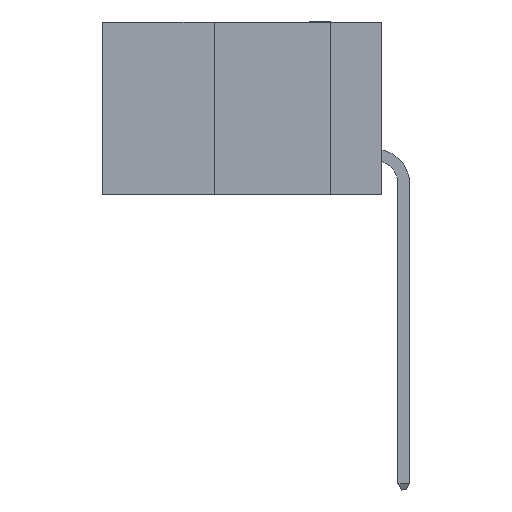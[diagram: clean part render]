
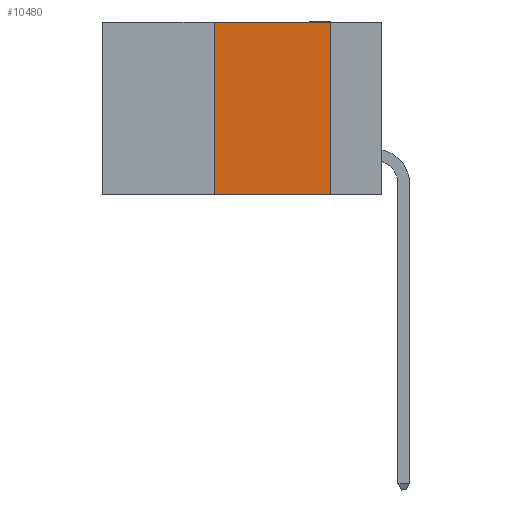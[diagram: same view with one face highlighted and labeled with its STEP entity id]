
A CAD part, left-side view. The second image highlights one B-rep face of the part: STEP entity #10480.
In plain terms, the highlighted planar face has unit normal (-1, 0, 0).
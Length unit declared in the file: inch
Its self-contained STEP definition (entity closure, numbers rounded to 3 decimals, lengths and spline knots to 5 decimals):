
#11 = ORIENTED_EDGE ( 'NONE', *, *, #4980, .F. ) ;
#479 = ORIENTED_EDGE ( 'NONE', *, *, #6891, .F. ) ;
#1325 = EDGE_CURVE ( 'NONE', #3748, #7478, #6699, .T. ) ;
#3245 = DIRECTION ( 'NONE',  ( 0., 0., -1. ) ) ;
#3409 = CARTESIAN_POINT ( 'NONE',  ( 0., 0.6, 0. ) ) ;
#3561 = CARTESIAN_POINT ( 'NONE',  ( 0., 0.11, 0. ) ) ;
#3644 = FACE_OUTER_BOUND ( 'NONE', #9182, .T. ) ;
#3748 = VERTEX_POINT ( 'NONE', #10097 ) ;
#4023 = VECTOR ( 'NONE', #10777, 39.37008 ) ;
#4320 = DIRECTION ( 'NONE',  ( 0., -1., 0. ) ) ;
#4980 = EDGE_CURVE ( 'NONE', #5077, #5996, #14956, .T. ) ;
#5077 = VERTEX_POINT ( 'NONE', #14675 ) ;
#5645 = LINE ( 'NONE', #6619, #14918 ) ;
#5758 = DIRECTION ( 'NONE',  ( 1., 0., 0. ) ) ;
#5996 = VERTEX_POINT ( 'NONE', #6702 ) ;
#6239 = VECTOR ( 'NONE', #14519, 39.37008 ) ;
#6619 = CARTESIAN_POINT ( 'NONE',  ( 0., 0.6, 0. ) ) ;
#6699 = LINE ( 'NONE', #3561, #4023 ) ;
#6702 = CARTESIAN_POINT ( 'NONE',  ( 0., 0.36, 0. ) ) ;
#6750 = CARTESIAN_POINT ( 'NONE',  ( 0., 0.11, -0.37 ) ) ;
#6891 = EDGE_CURVE ( 'NONE', #5996, #3748, #5645, .T. ) ;
#7478 = VERTEX_POINT ( 'NONE', #6750 ) ;
#7846 = CARTESIAN_POINT ( 'NONE',  ( 0., 0.6, -0.37 ) ) ;
#8190 = LINE ( 'NONE', #7846, #8388 ) ;
#8388 = VECTOR ( 'NONE', #10204, 39.37008 ) ;
#9182 = EDGE_LOOP ( 'NONE', ( #15441, #479, #11, #15531 ) ) ;
#10097 = CARTESIAN_POINT ( 'NONE',  ( 0., 0.11, 0. ) ) ;
#10204 = DIRECTION ( 'NONE',  ( 0., -1., 0. ) ) ;
#10480 = ADVANCED_FACE ( 'NONE', ( #3644 ), #10643, .F. ) ;
#10643 = PLANE ( 'NONE',  #12958 ) ;
#10777 = DIRECTION ( 'NONE',  ( 0., 0., -1. ) ) ;
#12958 = AXIS2_PLACEMENT_3D ( 'NONE', #3409, #5758, #3245 ) ;
#13322 = CARTESIAN_POINT ( 'NONE',  ( 0., 0.36, 0. ) ) ;
#14519 = DIRECTION ( 'NONE',  ( 0., 0., 1. ) ) ;
#14675 = CARTESIAN_POINT ( 'NONE',  ( 0., 0.36, -0.37 ) ) ;
#14918 = VECTOR ( 'NONE', #4320, 39.37008 ) ;
#14956 = LINE ( 'NONE', #13322, #6239 ) ;
#15441 = ORIENTED_EDGE ( 'NONE', *, *, #1325, .F. ) ;
#15521 = EDGE_CURVE ( 'NONE', #5077, #7478, #8190, .T. ) ;
#15531 = ORIENTED_EDGE ( 'NONE', *, *, #15521, .T. ) ;
